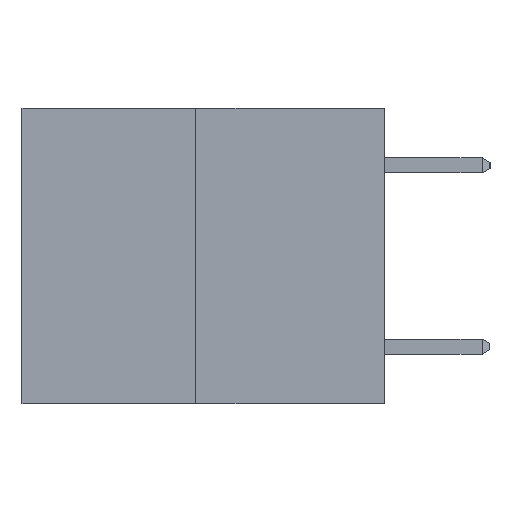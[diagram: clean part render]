
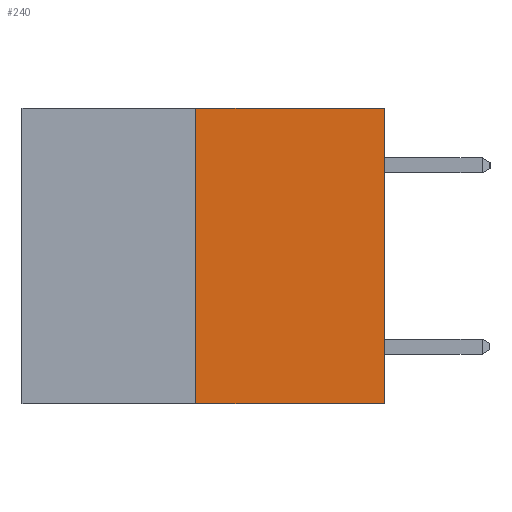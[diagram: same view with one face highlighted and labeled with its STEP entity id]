
A CAD part, left-side view. The second image highlights one B-rep face of the part: STEP entity #240.
In plain terms, the highlighted planar face has unit normal (-1, 0, 0).
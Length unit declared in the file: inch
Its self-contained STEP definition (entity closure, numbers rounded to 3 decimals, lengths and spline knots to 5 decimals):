
#64 = EDGE_CURVE ( 'NONE', #9649, #107, #7326, .T. ) ;
#107 = VERTEX_POINT ( 'NONE', #11275 ) ;
#185 = VERTEX_POINT ( 'NONE', #2512 ) ;
#240 = ADVANCED_FACE ( 'NONE', ( #10095 ), #6985, .F. ) ;
#863 = ORIENTED_EDGE ( 'NONE', *, *, #5624, .T. ) ;
#1040 = AXIS2_PLACEMENT_3D ( 'NONE', #6069, #10854, #9976 ) ;
#1571 = LINE ( 'NONE', #9763, #10817 ) ;
#2512 = CARTESIAN_POINT ( 'NONE',  ( 0., 0., 0. ) ) ;
#3145 = CARTESIAN_POINT ( 'NONE',  ( 0., 0.312, -0.49 ) ) ;
#3170 = ORIENTED_EDGE ( 'NONE', *, *, #4629, .T. ) ;
#3231 = VERTEX_POINT ( 'NONE', #7886 ) ;
#3274 = DIRECTION ( 'NONE',  ( 0., -1., 0. ) ) ;
#4584 = LINE ( 'NONE', #5102, #9046 ) ;
#4629 = EDGE_CURVE ( 'NONE', #3231, #185, #4584, .T. ) ;
#4977 = DIRECTION ( 'NONE',  ( 0., 0., 1. ) ) ;
#5102 = CARTESIAN_POINT ( 'NONE',  ( 0., 0., 0. ) ) ;
#5264 = EDGE_LOOP ( 'NONE', ( #9068, #863, #3170, #5620 ) ) ;
#5620 = ORIENTED_EDGE ( 'NONE', *, *, #7346, .F. ) ;
#5624 = EDGE_CURVE ( 'NONE', #9649, #3231, #10911, .T. ) ;
#6069 = CARTESIAN_POINT ( 'NONE',  ( 0., 0.6, 0. ) ) ;
#6768 = DIRECTION ( 'NONE',  ( 0., -1., 0. ) ) ;
#6885 = DIRECTION ( 'NONE',  ( 0., 0., 1. ) ) ;
#6985 = PLANE ( 'NONE',  #1040 ) ;
#7326 = LINE ( 'NONE', #7761, #9171 ) ;
#7346 = EDGE_CURVE ( 'NONE', #107, #185, #1571, .T. ) ;
#7761 = CARTESIAN_POINT ( 'NONE',  ( 0., 0.312, -0.49 ) ) ;
#7886 = CARTESIAN_POINT ( 'NONE',  ( 0., 0., -0.49 ) ) ;
#9046 = VECTOR ( 'NONE', #4977, 39.37008 ) ;
#9068 = ORIENTED_EDGE ( 'NONE', *, *, #64, .F. ) ;
#9171 = VECTOR ( 'NONE', #6885, 39.37008 ) ;
#9649 = VERTEX_POINT ( 'NONE', #3145 ) ;
#9763 = CARTESIAN_POINT ( 'NONE',  ( 0., 0.6, 0. ) ) ;
#9976 = DIRECTION ( 'NONE',  ( 0., 0., -1. ) ) ;
#10095 = FACE_OUTER_BOUND ( 'NONE', #5264, .T. ) ;
#10602 = VECTOR ( 'NONE', #3274, 39.37008 ) ;
#10817 = VECTOR ( 'NONE', #6768, 39.37008 ) ;
#10854 = DIRECTION ( 'NONE',  ( 1., 0., 0. ) ) ;
#10911 = LINE ( 'NONE', #11215, #10602 ) ;
#11215 = CARTESIAN_POINT ( 'NONE',  ( 0., 0.6, -0.49 ) ) ;
#11275 = CARTESIAN_POINT ( 'NONE',  ( 0., 0.312, 0. ) ) ;
